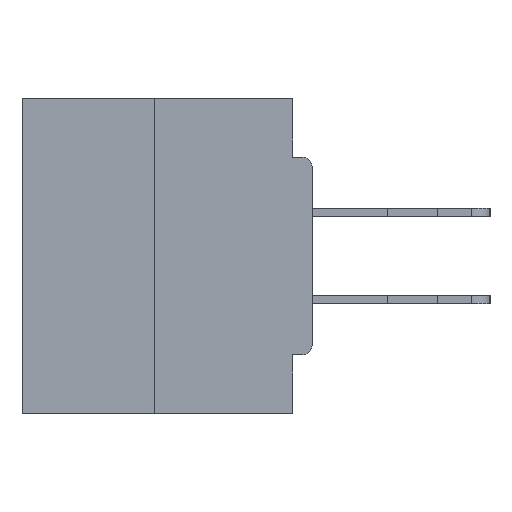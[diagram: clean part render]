
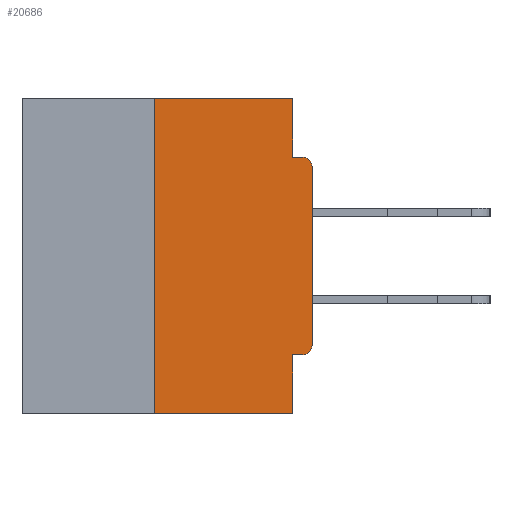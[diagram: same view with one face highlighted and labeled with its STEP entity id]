
A CAD part, left-side view. The second image highlights one B-rep face of the part: STEP entity #20686.
In plain terms, the highlighted planar face has unit normal (-1, 0, 0).
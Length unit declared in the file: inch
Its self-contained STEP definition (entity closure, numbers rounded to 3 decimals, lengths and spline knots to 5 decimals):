
#50 = VERTEX_POINT ( 'NONE', #7871 ) ;
#821 = VERTEX_POINT ( 'NONE', #4823 ) ;
#1080 = AXIS2_PLACEMENT_3D ( 'NONE', #12518, #36648, #18782 ) ;
#1538 = DIRECTION ( 'NONE',  ( 0., -1., 0. ) ) ;
#1911 = EDGE_CURVE ( 'NONE', #35794, #11011, #13326, .T. ) ;
#1973 = DIRECTION ( 'NONE',  ( 0., 1., 0. ) ) ;
#2557 = VECTOR ( 'NONE', #17904, 39.37008 ) ;
#2889 = ORIENTED_EDGE ( 'NONE', *, *, #28625, .F. ) ;
#3105 = CARTESIAN_POINT ( 'NONE',  ( 0., 0.46, -0.5 ) ) ;
#4075 = VERTEX_POINT ( 'NONE', #26793 ) ;
#4129 = EDGE_CURVE ( 'NONE', #34595, #27075, #20854, .T. ) ;
#4134 = EDGE_CURVE ( 'NONE', #20857, #8606, #18001, .T. ) ;
#4510 = CARTESIAN_POINT ( 'NONE',  ( 0., 0.031, -0.0935 ) ) ;
#4823 = CARTESIAN_POINT ( 'NONE',  ( 0., 0., -0.1085 ) ) ;
#6031 = ORIENTED_EDGE ( 'NONE', *, *, #12499, .T. ) ;
#6036 = ORIENTED_EDGE ( 'NONE', *, *, #4134, .T. ) ;
#6318 = CARTESIAN_POINT ( 'NONE',  ( 0., 0.031, 0. ) ) ;
#6763 = ORIENTED_EDGE ( 'NONE', *, *, #37388, .F. ) ;
#7136 = ORIENTED_EDGE ( 'NONE', *, *, #12913, .F. ) ;
#7871 = CARTESIAN_POINT ( 'NONE',  ( 0., 0.015, -0.0935 ) ) ;
#8195 = VECTOR ( 'NONE', #20478, 39.37008 ) ;
#8606 = VERTEX_POINT ( 'NONE', #28081 ) ;
#9104 = DIRECTION ( 'NONE',  ( 0., -1., 0. ) ) ;
#9374 = CARTESIAN_POINT ( 'NONE',  ( 0., 0., -0.0935 ) ) ;
#10195 = EDGE_CURVE ( 'NONE', #20857, #35794, #27961, .T. ) ;
#11011 = VERTEX_POINT ( 'NONE', #13476 ) ;
#11514 = LINE ( 'NONE', #23814, #34543 ) ;
#12499 = EDGE_CURVE ( 'NONE', #8606, #821, #27839, .T. ) ;
#12518 = CARTESIAN_POINT ( 'NONE',  ( 0., 0.015, -0.1085 ) ) ;
#12913 = EDGE_CURVE ( 'NONE', #27075, #50, #24968, .T. ) ;
#13326 = LINE ( 'NONE', #32501, #2557 ) ;
#13476 = CARTESIAN_POINT ( 'NONE',  ( 0., 0.031, -0.5 ) ) ;
#13570 = FACE_OUTER_BOUND ( 'NONE', #33469, .T. ) ;
#15652 = VECTOR ( 'NONE', #38474, 39.37008 ) ;
#16083 = EDGE_CURVE ( 'NONE', #16163, #11011, #24328, .T. ) ;
#16163 = VERTEX_POINT ( 'NONE', #28064 ) ;
#17904 = DIRECTION ( 'NONE',  ( 0., 0., -1. ) ) ;
#18001 = CIRCLE ( 'NONE', #20599, 0.015 ) ;
#18517 = ORIENTED_EDGE ( 'NONE', *, *, #1911, .F. ) ;
#18782 = DIRECTION ( 'NONE',  ( 0., 0., -1. ) ) ;
#19435 = AXIS2_PLACEMENT_3D ( 'NONE', #30090, #35984, #26924 ) ;
#20478 = DIRECTION ( 'NONE',  ( 0., 0., -1. ) ) ;
#20568 = CARTESIAN_POINT ( 'NONE',  ( 0., 0.015, -0.4065 ) ) ;
#20599 = AXIS2_PLACEMENT_3D ( 'NONE', #27060, #30239, #30097 ) ;
#20686 = ADVANCED_FACE ( 'NONE', ( #13570 ), #32987, .F. ) ;
#20854 = LINE ( 'NONE', #35477, #8195 ) ;
#20857 = VERTEX_POINT ( 'NONE', #20568 ) ;
#21997 = VECTOR ( 'NONE', #32999, 39.37008 ) ;
#23097 = CIRCLE ( 'NONE', #1080, 0.015 ) ;
#23814 = CARTESIAN_POINT ( 'NONE',  ( 0., 0.25, 0. ) ) ;
#24038 = VECTOR ( 'NONE', #1538, 39.37008 ) ;
#24198 = EDGE_CURVE ( 'NONE', #821, #50, #23097, .T. ) ;
#24328 = LINE ( 'NONE', #3105, #28529 ) ;
#24968 = LINE ( 'NONE', #9374, #24038 ) ;
#25133 = VECTOR ( 'NONE', #1973, 39.37008 ) ;
#25770 = ORIENTED_EDGE ( 'NONE', *, *, #24198, .T. ) ;
#26793 = CARTESIAN_POINT ( 'NONE',  ( 0., 0.25, 0. ) ) ;
#26924 = DIRECTION ( 'NONE',  ( 0., 0., -1. ) ) ;
#27060 = CARTESIAN_POINT ( 'NONE',  ( 0., 0.015, -0.3915 ) ) ;
#27075 = VERTEX_POINT ( 'NONE', #4510 ) ;
#27459 = CARTESIAN_POINT ( 'NONE',  ( 0., 0.46, 0. ) ) ;
#27839 = LINE ( 'NONE', #31299, #15652 ) ;
#27961 = LINE ( 'NONE', #31050, #25133 ) ;
#28064 = CARTESIAN_POINT ( 'NONE',  ( 0., 0.25, -0.5 ) ) ;
#28081 = CARTESIAN_POINT ( 'NONE',  ( 0., 0., -0.3915 ) ) ;
#28529 = VECTOR ( 'NONE', #9104, 39.37008 ) ;
#28625 = EDGE_CURVE ( 'NONE', #16163, #4075, #11514, .T. ) ;
#29453 = CARTESIAN_POINT ( 'NONE',  ( 0., 0.031, -0.4065 ) ) ;
#29514 = LINE ( 'NONE', #27459, #21997 ) ;
#30090 = CARTESIAN_POINT ( 'NONE',  ( 0., 0.46, 0. ) ) ;
#30097 = DIRECTION ( 'NONE',  ( 0., 0., -1. ) ) ;
#30239 = DIRECTION ( 'NONE',  ( -1., 0., 0. ) ) ;
#31050 = CARTESIAN_POINT ( 'NONE',  ( 0., 0., -0.4065 ) ) ;
#31083 = ORIENTED_EDGE ( 'NONE', *, *, #16083, .T. ) ;
#31299 = CARTESIAN_POINT ( 'NONE',  ( 0., 0., 0. ) ) ;
#32501 = CARTESIAN_POINT ( 'NONE',  ( 0., 0.031, -0.5 ) ) ;
#32977 = ORIENTED_EDGE ( 'NONE', *, *, #10195, .F. ) ;
#32987 = PLANE ( 'NONE',  #19435 ) ;
#32999 = DIRECTION ( 'NONE',  ( 0., -1., 0. ) ) ;
#33469 = EDGE_LOOP ( 'NONE', ( #6763, #2889, #31083, #18517, #32977, #6036, #6031, #25770, #7136, #34169 ) ) ;
#34169 = ORIENTED_EDGE ( 'NONE', *, *, #4129, .F. ) ;
#34543 = VECTOR ( 'NONE', #36051, 39.37008 ) ;
#34595 = VERTEX_POINT ( 'NONE', #6318 ) ;
#35477 = CARTESIAN_POINT ( 'NONE',  ( 0., 0.031, 0. ) ) ;
#35794 = VERTEX_POINT ( 'NONE', #29453 ) ;
#35984 = DIRECTION ( 'NONE',  ( 1., 0., 0. ) ) ;
#36051 = DIRECTION ( 'NONE',  ( 0., 0., 1. ) ) ;
#36648 = DIRECTION ( 'NONE',  ( -1., 0., 0. ) ) ;
#37388 = EDGE_CURVE ( 'NONE', #4075, #34595, #29514, .T. ) ;
#38474 = DIRECTION ( 'NONE',  ( 0., 0., 1. ) ) ;
